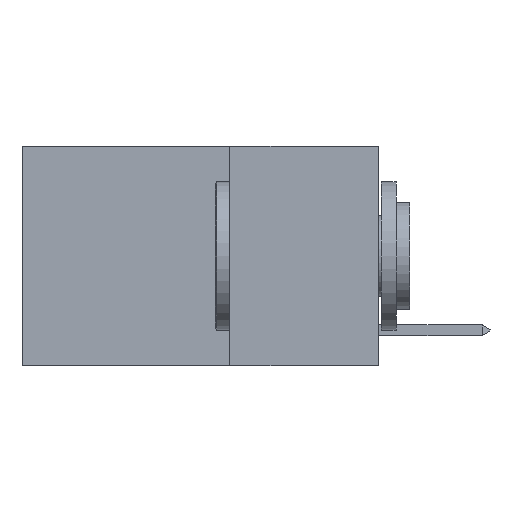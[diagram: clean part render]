
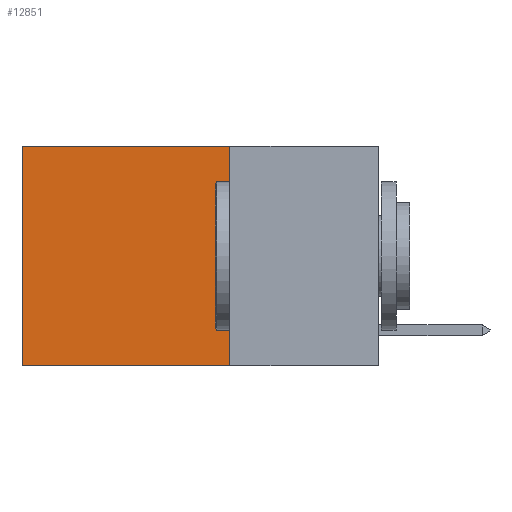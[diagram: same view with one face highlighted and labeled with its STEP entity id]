
A CAD part, left-side view. The second image highlights one B-rep face of the part: STEP entity #12851.
In plain terms, the highlighted planar face has unit normal (-1, 0, 0).
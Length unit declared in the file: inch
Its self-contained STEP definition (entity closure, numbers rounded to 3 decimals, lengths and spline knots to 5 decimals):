
#560 = VECTOR ( 'NONE', #11156, 39.37008 ) ;
#1792 = CARTESIAN_POINT ( 'NONE',  ( 0.2625, 0.6, 0. ) ) ;
#4448 = DIRECTION ( 'NONE',  ( 0., 0., -1. ) ) ;
#4531 = EDGE_LOOP ( 'NONE', ( #26618, #8025, #26863, #13932 ) ) ;
#5518 = CARTESIAN_POINT ( 'NONE',  ( 0.2625, 0.6, -0.37 ) ) ;
#5933 = CARTESIAN_POINT ( 'NONE',  ( 0.2625, 0.25, -0.37 ) ) ;
#6593 = CARTESIAN_POINT ( 'NONE',  ( 0.2625, 0.25, -0.37 ) ) ;
#7417 = EDGE_CURVE ( 'NONE', #10285, #20053, #26706, .T. ) ;
#8025 = ORIENTED_EDGE ( 'NONE', *, *, #14768, .F. ) ;
#8891 = CARTESIAN_POINT ( 'NONE',  ( 0.2625, 0.6, 0. ) ) ;
#8994 = DIRECTION ( 'NONE',  ( 0., 0., -1. ) ) ;
#10285 = VERTEX_POINT ( 'NONE', #1792 ) ;
#10762 = DIRECTION ( 'NONE',  ( 0., 0., -1. ) ) ;
#11009 = LINE ( 'NONE', #6593, #560 ) ;
#11156 = DIRECTION ( 'NONE',  ( 0., 1., 0. ) ) ;
#12148 = VECTOR ( 'NONE', #10762, 39.37008 ) ;
#12851 = ADVANCED_FACE ( 'NONE', ( #21656 ), #17457, .F. ) ;
#13932 = ORIENTED_EDGE ( 'NONE', *, *, #19713, .T. ) ;
#14768 = EDGE_CURVE ( 'NONE', #20749, #20053, #11009, .T. ) ;
#15600 = VECTOR ( 'NONE', #21346, 39.37008 ) ;
#17457 = PLANE ( 'NONE',  #26479 ) ;
#17742 = CARTESIAN_POINT ( 'NONE',  ( 0.2625, 0.25, 0. ) ) ;
#19396 = VECTOR ( 'NONE', #8994, 39.37008 ) ;
#19677 = CARTESIAN_POINT ( 'NONE',  ( 0.2625, 0.25, 0. ) ) ;
#19713 = EDGE_CURVE ( 'NONE', #27254, #10285, #26045, .T. ) ;
#20053 = VERTEX_POINT ( 'NONE', #5518 ) ;
#20749 = VERTEX_POINT ( 'NONE', #5933 ) ;
#21346 = DIRECTION ( 'NONE',  ( 0., 1., 0. ) ) ;
#21656 = FACE_OUTER_BOUND ( 'NONE', #4531, .T. ) ;
#24219 = EDGE_CURVE ( 'NONE', #27254, #20749, #27779, .T. ) ;
#24268 = DIRECTION ( 'NONE',  ( 1., 0., 0. ) ) ;
#25831 = CARTESIAN_POINT ( 'NONE',  ( 0.2625, 0.25, 0. ) ) ;
#26045 = LINE ( 'NONE', #25831, #15600 ) ;
#26116 = CARTESIAN_POINT ( 'NONE',  ( 0.2625, 0.25, 0. ) ) ;
#26479 = AXIS2_PLACEMENT_3D ( 'NONE', #19677, #24268, #4448 ) ;
#26618 = ORIENTED_EDGE ( 'NONE', *, *, #7417, .T. ) ;
#26706 = LINE ( 'NONE', #8891, #19396 ) ;
#26863 = ORIENTED_EDGE ( 'NONE', *, *, #24219, .F. ) ;
#27254 = VERTEX_POINT ( 'NONE', #17742 ) ;
#27779 = LINE ( 'NONE', #26116, #12148 ) ;
